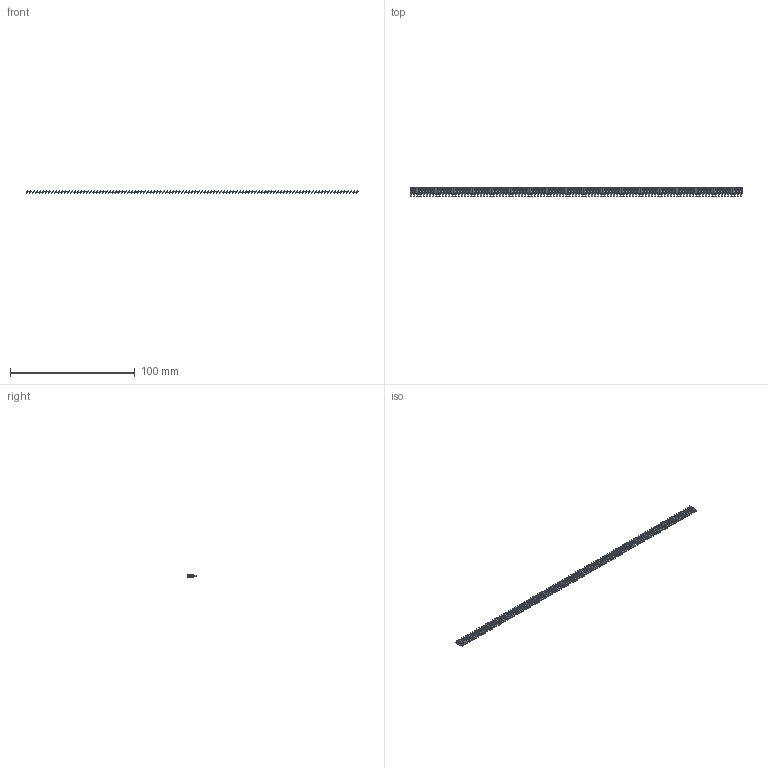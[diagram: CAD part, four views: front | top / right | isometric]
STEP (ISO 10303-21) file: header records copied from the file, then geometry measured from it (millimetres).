
FILE_DESCRIPTION (( 'STEP AP203' ), '1' );
FILE_NAME ('106-105-253-100.STEP', '2020-04-16T23:31:08', ( '' ), ( '' ), 'SwSTEP 2.0', 'SolidWorks 2016', '' );
FILE_SCHEMA (( 'CONFIG_CONTROL_DESIGN' ));
Length unit declared in the file: inch
Products named in the file (2): 100-290-001_100-290-253; 106-105-253-100
Assembly tree (105 placements, depth 2):
  106-105-253-100
    100-290-001_100-290-253  x105
Bounding box: 265.96 x 7.62 x 1.8 mm (x, y, z)
Volume: 579.3 mm3; surface area: 3612.7 mm2
Topology: 105 solids, 105 shells, 2100 faces, 5670 edges, 3780 vertices
Faces by surface type: plane 1995, cylinder 105
Entity records: 4148 total; most frequent: DIRECTION 312, CALENDAR_DATE 220, COORDINATED_UNIVERSAL_TIME_OFFSET 220, DATE_AND_TIME 220, LOCAL_TIME 220, CARTESIAN_POINT 218, AXIS2_PLACEMENT_3D 130, PERSON_AND_ORGANIZATION 121
